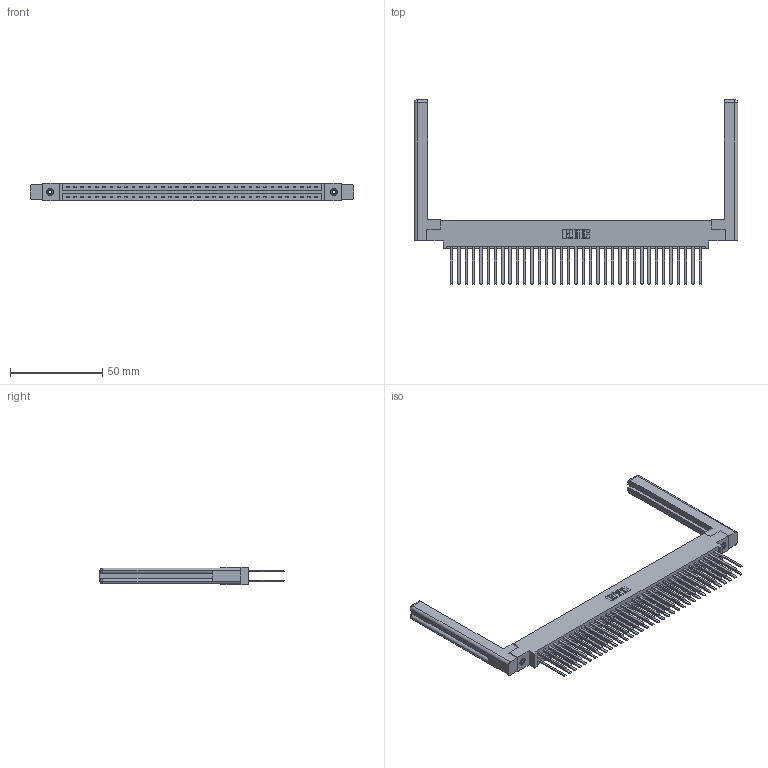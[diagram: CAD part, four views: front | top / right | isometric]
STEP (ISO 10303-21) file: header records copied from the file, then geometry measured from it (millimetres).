
FILE_DESCRIPTION (( 'STEP AP203' ), '1' );
FILE_NAME ('337-070-544-858.STEP', '2019-10-15T11:05:51', ( '' ), ( '' ), 'SwSTEP 2.0', 'SolidWorks 2016', '' );
FILE_SCHEMA (( 'CONFIG_CONTROL_DESIGN' ));
Length unit declared in the file: inch
Products named in the file (5): 337-070-544-858; 337 Part_0.170 Offset - 0.156 Dia-TI; 345-292-001_345-293-144; 307-220-058; 345-250-001_345-250-001-102
Assembly tree (75 placements, depth 2):
  337-070-544-858
    337 Part_0.170 Offset - 0.156 Dia-TI
    345-292-001_345-293-144  x70
    345-250-001_345-250-001-102  x2
    307-220-058  x2
Bounding box: 175.31 x 99.7 x 9.4 mm (x, y, z)
Volume: 26388.6 mm3; surface area: 30050 mm2
Topology: 75 solids, 75 shells, 3620 faces, 10687 edges, 7018 vertices
Faces by surface type: plane 2538, cylinder 1058, cone 12, torus 12
Entity records: 30624 total; most frequent: CARTESIAN_POINT 5173, ORIENTED_EDGE 5048, DIRECTION 4424, EDGE_CURVE 2524, LINE 2352, VECTOR 2352, VERTEX_POINT 1674, AXIS2_PLACEMENT_3D 1036
